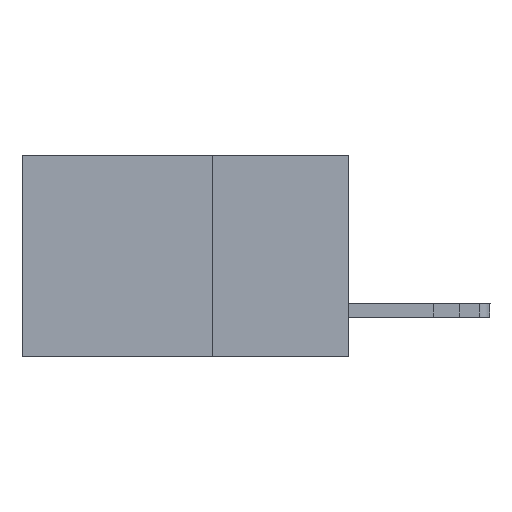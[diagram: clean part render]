
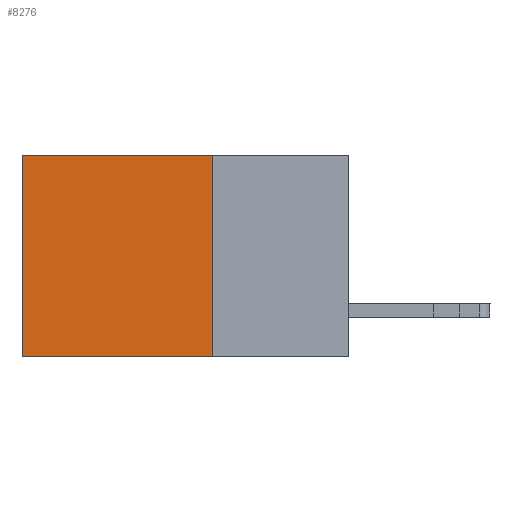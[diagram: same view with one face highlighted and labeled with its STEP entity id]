
A CAD part, left-side view. The second image highlights one B-rep face of the part: STEP entity #8276.
In plain terms, the highlighted planar face has unit normal (-1, 0, 0).
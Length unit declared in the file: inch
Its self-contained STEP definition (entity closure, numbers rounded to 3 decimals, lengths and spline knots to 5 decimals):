
#466 = VERTEX_POINT ( 'NONE', #3385 ) ;
#677 = ORIENTED_EDGE ( 'NONE', *, *, #9209, .F. ) ;
#968 = CARTESIAN_POINT ( 'NONE',  ( 0.2615, 0.6, -0.37 ) ) ;
#1869 = EDGE_CURVE ( 'NONE', #9912, #466, #5626, .T. ) ;
#1963 = CARTESIAN_POINT ( 'NONE',  ( 0.2615, 0.25, -0.37 ) ) ;
#2042 = EDGE_CURVE ( 'NONE', #9912, #8307, #2960, .T. ) ;
#2154 = FACE_OUTER_BOUND ( 'NONE', #8823, .T. ) ;
#2331 = VERTEX_POINT ( 'NONE', #6068 ) ;
#2526 = LINE ( 'NONE', #968, #7192 ) ;
#2960 = LINE ( 'NONE', #9835, #7538 ) ;
#3253 = VECTOR ( 'NONE', #7164, 39.37008 ) ;
#3385 = CARTESIAN_POINT ( 'NONE',  ( 0.2615, 0.25, -0.37 ) ) ;
#4108 = DIRECTION ( 'NONE',  ( 0., 0., -1. ) ) ;
#4360 = AXIS2_PLACEMENT_3D ( 'NONE', #9191, #6206, #8374 ) ;
#4527 = DIRECTION ( 'NONE',  ( 0., 1., 0. ) ) ;
#4660 = PLANE ( 'NONE',  #4360 ) ;
#4848 = ORIENTED_EDGE ( 'NONE', *, *, #2042, .T. ) ;
#5156 = DIRECTION ( 'NONE',  ( 0., 1., 0. ) ) ;
#5244 = ORIENTED_EDGE ( 'NONE', *, *, #1869, .F. ) ;
#5626 = LINE ( 'NONE', #1963, #3253 ) ;
#6068 = CARTESIAN_POINT ( 'NONE',  ( 0.2615, 0.6, -0.37 ) ) ;
#6206 = DIRECTION ( 'NONE',  ( 1., 0., 0. ) ) ;
#7164 = DIRECTION ( 'NONE',  ( 0., 0., -1. ) ) ;
#7192 = VECTOR ( 'NONE', #4108, 39.37008 ) ;
#7538 = VECTOR ( 'NONE', #5156, 39.37008 ) ;
#7556 = CARTESIAN_POINT ( 'NONE',  ( 0.2615, 0.25, 0. ) ) ;
#8276 = ADVANCED_FACE ( 'NONE', ( #2154 ), #4660, .F. ) ;
#8307 = VERTEX_POINT ( 'NONE', #9405 ) ;
#8374 = DIRECTION ( 'NONE',  ( 0., 0., -1. ) ) ;
#8823 = EDGE_LOOP ( 'NONE', ( #8987, #677, #5244, #4848 ) ) ;
#8987 = ORIENTED_EDGE ( 'NONE', *, *, #9852, .T. ) ;
#9191 = CARTESIAN_POINT ( 'NONE',  ( 0.2615, 0.25, -0.37 ) ) ;
#9209 = EDGE_CURVE ( 'NONE', #466, #2331, #10082, .T. ) ;
#9312 = CARTESIAN_POINT ( 'NONE',  ( 0.2615, 0.25, -0.37 ) ) ;
#9405 = CARTESIAN_POINT ( 'NONE',  ( 0.2615, 0.6, 0. ) ) ;
#9628 = VECTOR ( 'NONE', #4527, 39.37008 ) ;
#9835 = CARTESIAN_POINT ( 'NONE',  ( 0.2615, 0.25, 0. ) ) ;
#9852 = EDGE_CURVE ( 'NONE', #8307, #2331, #2526, .T. ) ;
#9912 = VERTEX_POINT ( 'NONE', #7556 ) ;
#10082 = LINE ( 'NONE', #9312, #9628 ) ;
